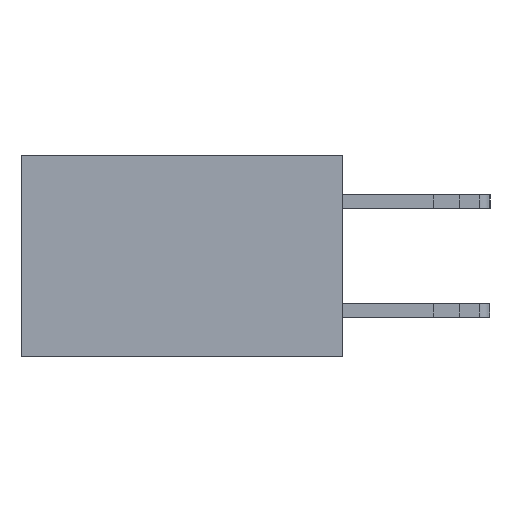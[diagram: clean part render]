
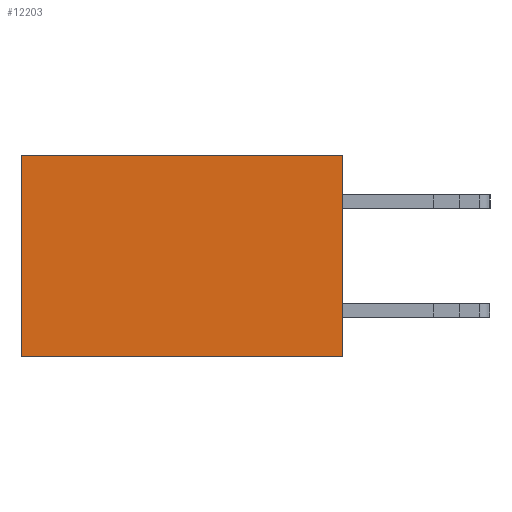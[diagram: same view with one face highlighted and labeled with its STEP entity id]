
A CAD part, left-side view. The second image highlights one B-rep face of the part: STEP entity #12203.
In plain terms, the highlighted planar face has unit normal (-1, 0, 0).
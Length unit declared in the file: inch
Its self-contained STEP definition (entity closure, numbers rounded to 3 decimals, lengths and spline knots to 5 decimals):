
#590 = LINE ( 'NONE', #17517, #18093 ) ;
#763 = CARTESIAN_POINT ( 'NONE',  ( 0.277, 0., -0.37 ) ) ;
#987 = VERTEX_POINT ( 'NONE', #16786 ) ;
#2790 = DIRECTION ( 'NONE',  ( 0., 0., -1. ) ) ;
#3695 = CARTESIAN_POINT ( 'NONE',  ( 0.277, 0.59, -0.37 ) ) ;
#4947 = AXIS2_PLACEMENT_3D ( 'NONE', #763, #7344, #21948 ) ;
#4971 = CARTESIAN_POINT ( 'NONE',  ( 0.277, 0., -0.37 ) ) ;
#5024 = CARTESIAN_POINT ( 'NONE',  ( 0.277, 0., 0. ) ) ;
#6401 = ORIENTED_EDGE ( 'NONE', *, *, #16711, .F. ) ;
#7112 = DIRECTION ( 'NONE',  ( 0., 1., 0. ) ) ;
#7344 = DIRECTION ( 'NONE',  ( 1., 0., 0. ) ) ;
#9532 = ORIENTED_EDGE ( 'NONE', *, *, #17456, .T. ) ;
#9815 = VECTOR ( 'NONE', #7112, 39.37008 ) ;
#10273 = VECTOR ( 'NONE', #23719, 39.37008 ) ;
#10478 = LINE ( 'NONE', #4971, #9815 ) ;
#12136 = VERTEX_POINT ( 'NONE', #23716 ) ;
#12203 = ADVANCED_FACE ( 'NONE', ( #21913 ), #19843, .F. ) ;
#12417 = VERTEX_POINT ( 'NONE', #3695 ) ;
#12664 = VERTEX_POINT ( 'NONE', #13064 ) ;
#13064 = CARTESIAN_POINT ( 'NONE',  ( 0.277, 0., -0.37 ) ) ;
#13427 = EDGE_CURVE ( 'NONE', #12664, #12417, #10478, .T. ) ;
#14133 = CARTESIAN_POINT ( 'NONE',  ( 0.277, 0.59, -0.37 ) ) ;
#15307 = ORIENTED_EDGE ( 'NONE', *, *, #13427, .F. ) ;
#16711 = EDGE_CURVE ( 'NONE', #12136, #12664, #590, .T. ) ;
#16786 = CARTESIAN_POINT ( 'NONE',  ( 0.277, 0.59, 0. ) ) ;
#17456 = EDGE_CURVE ( 'NONE', #12136, #987, #21971, .T. ) ;
#17517 = CARTESIAN_POINT ( 'NONE',  ( 0.277, 0., -0.37 ) ) ;
#17691 = EDGE_LOOP ( 'NONE', ( #18826, #15307, #6401, #9532 ) ) ;
#17819 = VECTOR ( 'NONE', #18177, 39.37008 ) ;
#18093 = VECTOR ( 'NONE', #2790, 39.37008 ) ;
#18177 = DIRECTION ( 'NONE',  ( 0., 0., -1. ) ) ;
#18826 = ORIENTED_EDGE ( 'NONE', *, *, #26487, .T. ) ;
#19843 = PLANE ( 'NONE',  #4947 ) ;
#21913 = FACE_OUTER_BOUND ( 'NONE', #17691, .T. ) ;
#21948 = DIRECTION ( 'NONE',  ( 0., 0., -1. ) ) ;
#21971 = LINE ( 'NONE', #5024, #10273 ) ;
#22693 = LINE ( 'NONE', #14133, #17819 ) ;
#23716 = CARTESIAN_POINT ( 'NONE',  ( 0.277, 0., 0. ) ) ;
#23719 = DIRECTION ( 'NONE',  ( 0., 1., 0. ) ) ;
#26487 = EDGE_CURVE ( 'NONE', #987, #12417, #22693, .T. ) ;
